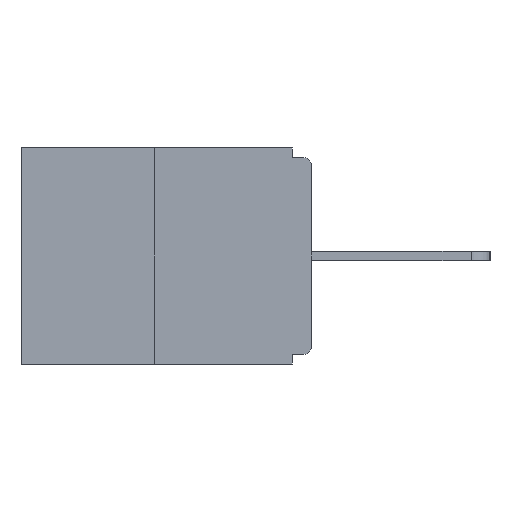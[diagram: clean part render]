
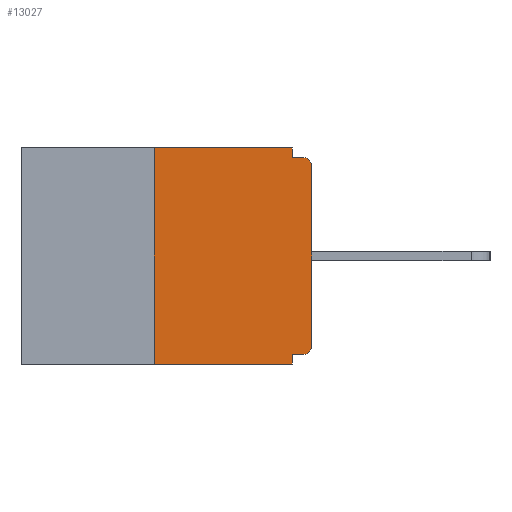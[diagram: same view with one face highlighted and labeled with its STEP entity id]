
A CAD part, left-side view. The second image highlights one B-rep face of the part: STEP entity #13027.
In plain terms, the highlighted planar face has unit normal (-1, 0, 0).
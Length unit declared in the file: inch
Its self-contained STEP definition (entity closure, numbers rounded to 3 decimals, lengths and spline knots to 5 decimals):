
#26 = DIRECTION ( 'NONE',  ( 1., 0., 0. ) ) ;
#178 = DIRECTION ( 'NONE',  ( 0., 0., 1. ) ) ;
#247 = VERTEX_POINT ( 'NONE', #19974 ) ;
#264 = ORIENTED_EDGE ( 'NONE', *, *, #15073, .F. ) ;
#416 = EDGE_CURVE ( 'NONE', #18436, #247, #13011, .T. ) ;
#708 = LINE ( 'NONE', #5264, #12403 ) ;
#2096 = ORIENTED_EDGE ( 'NONE', *, *, #17715, .T. ) ;
#2244 = VECTOR ( 'NONE', #12579, 39.37008 ) ;
#2307 = CARTESIAN_POINT ( 'NONE',  ( 0., 0.25, -0.343 ) ) ;
#3050 = CARTESIAN_POINT ( 'NONE',  ( 0., 0.46, 0. ) ) ;
#3131 = CARTESIAN_POINT ( 'NONE',  ( 0., 0.015, -0.03 ) ) ;
#3195 = VECTOR ( 'NONE', #17571, 39.37008 ) ;
#3280 = ORIENTED_EDGE ( 'NONE', *, *, #12651, .F. ) ;
#3309 = CARTESIAN_POINT ( 'NONE',  ( 0., 0.25, 0. ) ) ;
#3406 = DIRECTION ( 'NONE',  ( 0., 1., 0. ) ) ;
#3945 = CARTESIAN_POINT ( 'NONE',  ( 0., 0.46, 0. ) ) ;
#4480 = VERTEX_POINT ( 'NONE', #8470 ) ;
#4491 = DIRECTION ( 'NONE',  ( 0., 0., -1. ) ) ;
#4736 = DIRECTION ( 'NONE',  ( -1., 0., 0. ) ) ;
#4743 = CARTESIAN_POINT ( 'NONE',  ( 0., 0.015, -0.015 ) ) ;
#4951 = LINE ( 'NONE', #3309, #15718 ) ;
#5264 = CARTESIAN_POINT ( 'NONE',  ( 0., 0.46, -0.343 ) ) ;
#5449 = CARTESIAN_POINT ( 'NONE',  ( 0., 0.031, -0.328 ) ) ;
#5494 = CARTESIAN_POINT ( 'NONE',  ( 0., 0.031, -0.015 ) ) ;
#5627 = VERTEX_POINT ( 'NONE', #4743 ) ;
#5868 = VECTOR ( 'NONE', #3406, 39.37008 ) ;
#6125 = CARTESIAN_POINT ( 'NONE',  ( 0., 0.031, 0. ) ) ;
#6573 = CARTESIAN_POINT ( 'NONE',  ( 0., 0., -0.313 ) ) ;
#6682 = EDGE_CURVE ( 'NONE', #16664, #5627, #17616, .T. ) ;
#6740 = VERTEX_POINT ( 'NONE', #13275 ) ;
#7125 = CIRCLE ( 'NONE', #9093, 0.015 ) ;
#7720 = CARTESIAN_POINT ( 'NONE',  ( 0., 0., -0.015 ) ) ;
#7957 = CARTESIAN_POINT ( 'NONE',  ( 0., 0., -0.03 ) ) ;
#8057 = DIRECTION ( 'NONE',  ( 0., 0., -1. ) ) ;
#8154 = CARTESIAN_POINT ( 'NONE',  ( 0., 0., -0.328 ) ) ;
#8385 = LINE ( 'NONE', #3945, #14535 ) ;
#8470 = CARTESIAN_POINT ( 'NONE',  ( 0., 0.015, -0.328 ) ) ;
#8573 = ORIENTED_EDGE ( 'NONE', *, *, #416, .F. ) ;
#9075 = LINE ( 'NONE', #15414, #10870 ) ;
#9093 = AXIS2_PLACEMENT_3D ( 'NONE', #17303, #4736, #8057 ) ;
#9173 = EDGE_LOOP ( 'NONE', ( #264, #17554, #12998, #8573, #12540, #2096, #17502, #19204, #3280, #15154 ) ) ;
#10870 = VECTOR ( 'NONE', #20264, 39.37008 ) ;
#11561 = DIRECTION ( 'NONE',  ( 0., -1., 0. ) ) ;
#11745 = VERTEX_POINT ( 'NONE', #2307 ) ;
#12403 = VECTOR ( 'NONE', #11561, 39.37008 ) ;
#12540 = ORIENTED_EDGE ( 'NONE', *, *, #13433, .F. ) ;
#12579 = DIRECTION ( 'NONE',  ( 0., -1., 0. ) ) ;
#12647 = DIRECTION ( 'NONE',  ( 0., 0., -1. ) ) ;
#12651 = EDGE_CURVE ( 'NONE', #15094, #5627, #17369, .T. ) ;
#12694 = EDGE_CURVE ( 'NONE', #19992, #16664, #12780, .T. ) ;
#12780 = LINE ( 'NONE', #19119, #3195 ) ;
#12921 = LINE ( 'NONE', #8154, #5868 ) ;
#12998 = ORIENTED_EDGE ( 'NONE', *, *, #17826, .T. ) ;
#13011 = LINE ( 'NONE', #19340, #20383 ) ;
#13027 = ADVANCED_FACE ( 'NONE', ( #15987 ), #15783, .F. ) ;
#13275 = CARTESIAN_POINT ( 'NONE',  ( 0., 0.25, 0. ) ) ;
#13433 = EDGE_CURVE ( 'NONE', #4480, #18436, #12921, .T. ) ;
#14117 = AXIS2_PLACEMENT_3D ( 'NONE', #3050, #26, #4491 ) ;
#14269 = DIRECTION ( 'NONE',  ( 0., 0., -1. ) ) ;
#14535 = VECTOR ( 'NONE', #16172, 39.37008 ) ;
#15073 = EDGE_CURVE ( 'NONE', #6740, #19088, #8385, .T. ) ;
#15094 = VERTEX_POINT ( 'NONE', #5494 ) ;
#15154 = ORIENTED_EDGE ( 'NONE', *, *, #15268, .F. ) ;
#15268 = EDGE_CURVE ( 'NONE', #19088, #15094, #9075, .T. ) ;
#15414 = CARTESIAN_POINT ( 'NONE',  ( 0., 0.031, 0. ) ) ;
#15678 = DIRECTION ( 'NONE',  ( -1., 0., 0. ) ) ;
#15718 = VECTOR ( 'NONE', #178, 39.37008 ) ;
#15783 = PLANE ( 'NONE',  #14117 ) ;
#15987 = FACE_OUTER_BOUND ( 'NONE', #9173, .T. ) ;
#16172 = DIRECTION ( 'NONE',  ( 0., -1., 0. ) ) ;
#16284 = AXIS2_PLACEMENT_3D ( 'NONE', #3131, #15678, #12647 ) ;
#16664 = VERTEX_POINT ( 'NONE', #7957 ) ;
#17303 = CARTESIAN_POINT ( 'NONE',  ( 0., 0.015, -0.313 ) ) ;
#17369 = LINE ( 'NONE', #7720, #2244 ) ;
#17502 = ORIENTED_EDGE ( 'NONE', *, *, #12694, .T. ) ;
#17554 = ORIENTED_EDGE ( 'NONE', *, *, #17735, .F. ) ;
#17571 = DIRECTION ( 'NONE',  ( 0., 0., 1. ) ) ;
#17616 = CIRCLE ( 'NONE', #16284, 0.015 ) ;
#17715 = EDGE_CURVE ( 'NONE', #4480, #19992, #7125, .T. ) ;
#17735 = EDGE_CURVE ( 'NONE', #11745, #6740, #4951, .T. ) ;
#17826 = EDGE_CURVE ( 'NONE', #11745, #247, #708, .T. ) ;
#18436 = VERTEX_POINT ( 'NONE', #5449 ) ;
#19088 = VERTEX_POINT ( 'NONE', #6125 ) ;
#19119 = CARTESIAN_POINT ( 'NONE',  ( 0., 0., 0. ) ) ;
#19204 = ORIENTED_EDGE ( 'NONE', *, *, #6682, .T. ) ;
#19340 = CARTESIAN_POINT ( 'NONE',  ( 0., 0.031, -0.343 ) ) ;
#19974 = CARTESIAN_POINT ( 'NONE',  ( 0., 0.031, -0.343 ) ) ;
#19992 = VERTEX_POINT ( 'NONE', #6573 ) ;
#20264 = DIRECTION ( 'NONE',  ( 0., 0., -1. ) ) ;
#20383 = VECTOR ( 'NONE', #14269, 39.37008 ) ;
